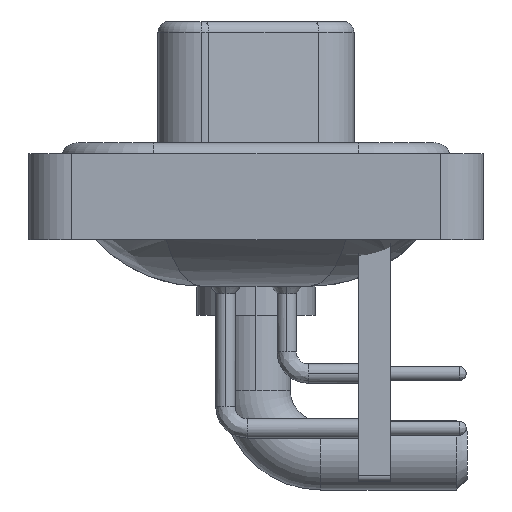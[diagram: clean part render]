
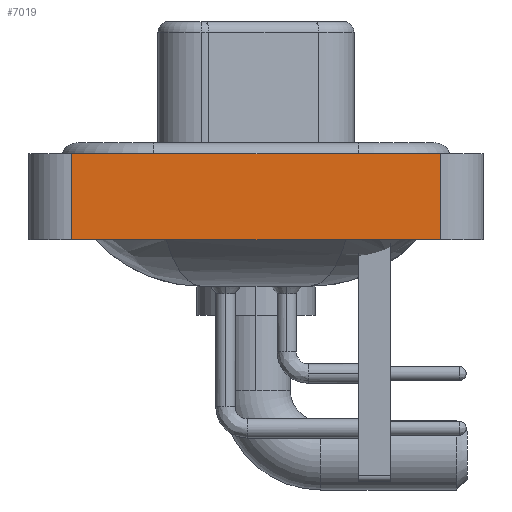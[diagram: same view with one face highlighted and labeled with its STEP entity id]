
A CAD part, left-side view. The second image highlights one B-rep face of the part: STEP entity #7019.
In plain terms, the highlighted planar face has unit normal (-1, 0, 0).
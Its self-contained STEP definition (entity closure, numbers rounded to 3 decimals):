
#1777 = CARTESIAN_POINT ( 'NONE',  ( -7.35, 8.55, -3.6 ) ) ;
#1880 = CARTESIAN_POINT ( 'NONE',  ( -7.35, -8.55, -3.6 ) ) ;
#2223 = EDGE_CURVE ( 'NONE', #18073, #19391, #25897, .T. ) ;
#3277 = EDGE_CURVE ( 'NONE', #12629, #18073, #11143, .T. ) ;
#6732 = ORIENTED_EDGE ( 'NONE', *, *, #2223, .F. ) ;
#7019 = ADVANCED_FACE ( 'NONE', ( #27264 ), #16039, .T. ) ;
#8540 = DIRECTION ( 'NONE',  ( -1., 0., 0. ) ) ;
#8671 = LINE ( 'NONE', #25243, #12824 ) ;
#8781 = LINE ( 'NONE', #1880, #23895 ) ;
#9372 = EDGE_CURVE ( 'NONE', #13376, #19391, #8671, .T. ) ;
#10847 = DIRECTION ( 'NONE',  ( 0., 0., 1. ) ) ;
#11143 = LINE ( 'NONE', #1777, #15980 ) ;
#12410 = ORIENTED_EDGE ( 'NONE', *, *, #9372, .T. ) ;
#12629 = VERTEX_POINT ( 'NONE', #27318 ) ;
#12824 = VECTOR ( 'NONE', #18190, 1000. ) ;
#13092 = DIRECTION ( 'NONE',  ( 0., -1., 0. ) ) ;
#13376 = VERTEX_POINT ( 'NONE', #22193 ) ;
#13874 = CARTESIAN_POINT ( 'NONE',  ( -7.35, -8.55, -3.6 ) ) ;
#14499 = ORIENTED_EDGE ( 'NONE', *, *, #25211, .T. ) ;
#15980 = VECTOR ( 'NONE', #22357, 1000. ) ;
#16000 = AXIS2_PLACEMENT_3D ( 'NONE', #13874, #8540, #10847 ) ;
#16039 = PLANE ( 'NONE',  #16000 ) ;
#18073 = VERTEX_POINT ( 'NONE', #23875 ) ;
#18190 = DIRECTION ( 'NONE',  ( 0., 0., 1. ) ) ;
#19308 = CARTESIAN_POINT ( 'NONE',  ( -7.35, -8.55, 0.4 ) ) ;
#19391 = VERTEX_POINT ( 'NONE', #28505 ) ;
#22193 = CARTESIAN_POINT ( 'NONE',  ( -7.35, -8.55, -3.6 ) ) ;
#22357 = DIRECTION ( 'NONE',  ( 0., 0., 1. ) ) ;
#23875 = CARTESIAN_POINT ( 'NONE',  ( -7.35, 8.55, 0.4 ) ) ;
#23895 = VECTOR ( 'NONE', #13092, 1000. ) ;
#24742 = VECTOR ( 'NONE', #26347, 1000. ) ;
#25211 = EDGE_CURVE ( 'NONE', #12629, #13376, #8781, .T. ) ;
#25243 = CARTESIAN_POINT ( 'NONE',  ( -7.35, -8.55, -3.6 ) ) ;
#25897 = LINE ( 'NONE', #19308, #24742 ) ;
#26347 = DIRECTION ( 'NONE',  ( 0., -1., 0. ) ) ;
#27213 = ORIENTED_EDGE ( 'NONE', *, *, #3277, .F. ) ;
#27264 = FACE_OUTER_BOUND ( 'NONE', #29921, .T. ) ;
#27318 = CARTESIAN_POINT ( 'NONE',  ( -7.35, 8.55, -3.6 ) ) ;
#28505 = CARTESIAN_POINT ( 'NONE',  ( -7.35, -8.55, 0.4 ) ) ;
#29921 = EDGE_LOOP ( 'NONE', ( #12410, #6732, #27213, #14499 ) ) ;
